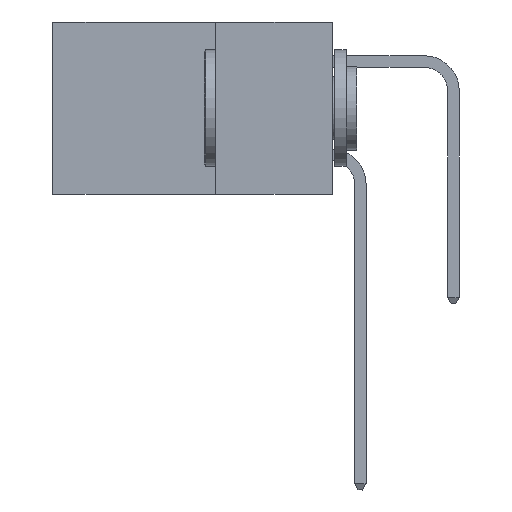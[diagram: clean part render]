
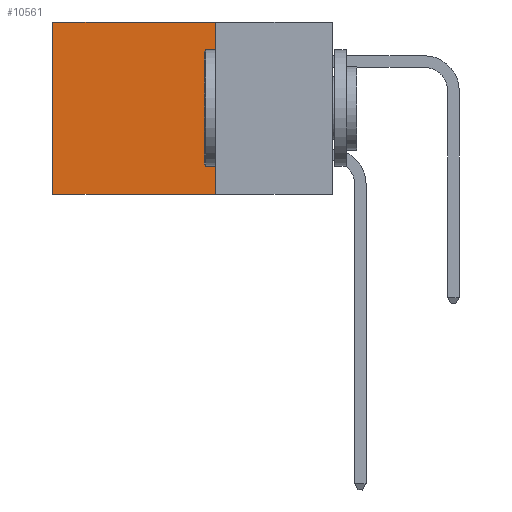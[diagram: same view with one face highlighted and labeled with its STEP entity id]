
A CAD part, left-side view. The second image highlights one B-rep face of the part: STEP entity #10561.
In plain terms, the highlighted planar face has unit normal (-1, 0, 0).
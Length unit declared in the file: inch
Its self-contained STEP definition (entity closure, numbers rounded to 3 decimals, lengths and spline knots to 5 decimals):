
#66 = VECTOR ( 'NONE', #5421, 39.37008 ) ;
#1281 = VERTEX_POINT ( 'NONE', #7742 ) ;
#1381 = ORIENTED_EDGE ( 'NONE', *, *, #11467, .T. ) ;
#1553 = CARTESIAN_POINT ( 'NONE',  ( 0.298, 0.25, 0. ) ) ;
#1686 = VECTOR ( 'NONE', #6992, 39.37008 ) ;
#2021 = PLANE ( 'NONE',  #2834 ) ;
#2365 = CARTESIAN_POINT ( 'NONE',  ( 0.298, 0.6, -0.37 ) ) ;
#2624 = LINE ( 'NONE', #10029, #66 ) ;
#2743 = LINE ( 'NONE', #7984, #1686 ) ;
#2834 = AXIS2_PLACEMENT_3D ( 'NONE', #4071, #6919, #6835 ) ;
#3186 = VERTEX_POINT ( 'NONE', #2365 ) ;
#4071 = CARTESIAN_POINT ( 'NONE',  ( 0.298, 0.25, 0. ) ) ;
#4366 = CARTESIAN_POINT ( 'NONE',  ( 0.298, 0.6, 0. ) ) ;
#4849 = EDGE_CURVE ( 'NONE', #1281, #3186, #8381, .T. ) ;
#5421 = DIRECTION ( 'NONE',  ( 0., 1., 0. ) ) ;
#6142 = ORIENTED_EDGE ( 'NONE', *, *, #4849, .T. ) ;
#6245 = VECTOR ( 'NONE', #11957, 39.37008 ) ;
#6335 = ORIENTED_EDGE ( 'NONE', *, *, #7762, .F. ) ;
#6835 = DIRECTION ( 'NONE',  ( 0., 0., -1. ) ) ;
#6919 = DIRECTION ( 'NONE',  ( 1., 0., 0. ) ) ;
#6992 = DIRECTION ( 'NONE',  ( 0., 1., 0. ) ) ;
#7742 = CARTESIAN_POINT ( 'NONE',  ( 0.298, 0.6, 0. ) ) ;
#7762 = EDGE_CURVE ( 'NONE', #11624, #9953, #12129, .T. ) ;
#7984 = CARTESIAN_POINT ( 'NONE',  ( 0.298, 0.25, 0. ) ) ;
#8381 = LINE ( 'NONE', #4366, #9589 ) ;
#8433 = CARTESIAN_POINT ( 'NONE',  ( 0.298, 0.25, -0.37 ) ) ;
#9210 = EDGE_LOOP ( 'NONE', ( #6142, #9586, #6335, #1381 ) ) ;
#9586 = ORIENTED_EDGE ( 'NONE', *, *, #10702, .F. ) ;
#9589 = VECTOR ( 'NONE', #10269, 39.37008 ) ;
#9953 = VERTEX_POINT ( 'NONE', #8433 ) ;
#10029 = CARTESIAN_POINT ( 'NONE',  ( 0.298, 0.25, -0.37 ) ) ;
#10254 = CARTESIAN_POINT ( 'NONE',  ( 0.298, 0.25, 0. ) ) ;
#10269 = DIRECTION ( 'NONE',  ( 0., 0., -1. ) ) ;
#10561 = ADVANCED_FACE ( 'NONE', ( #10866 ), #2021, .F. ) ;
#10702 = EDGE_CURVE ( 'NONE', #9953, #3186, #2624, .T. ) ;
#10866 = FACE_OUTER_BOUND ( 'NONE', #9210, .T. ) ;
#11467 = EDGE_CURVE ( 'NONE', #11624, #1281, #2743, .T. ) ;
#11624 = VERTEX_POINT ( 'NONE', #10254 ) ;
#11957 = DIRECTION ( 'NONE',  ( 0., 0., -1. ) ) ;
#12129 = LINE ( 'NONE', #1553, #6245 ) ;
